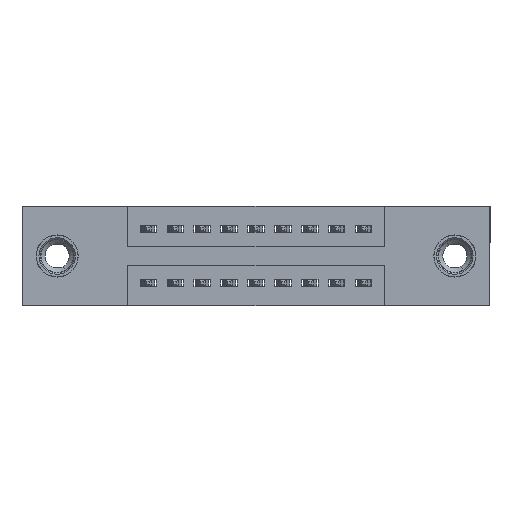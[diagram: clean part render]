
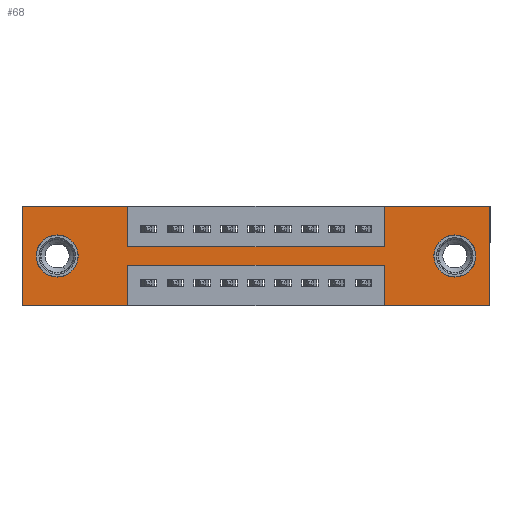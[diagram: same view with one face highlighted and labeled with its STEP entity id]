
A CAD part, front view. The second image highlights one B-rep face of the part: STEP entity #68.
In plain terms, the highlighted planar face has unit normal (0, -1, 0).
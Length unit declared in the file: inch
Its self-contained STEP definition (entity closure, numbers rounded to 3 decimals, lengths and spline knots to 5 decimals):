
#68 = ADVANCED_FACE ( 'NONE', ( #8803, #8489, #3202 ), #11013, .T. ) ;
#75 = VECTOR ( 'NONE', #6077, 39.37008 ) ;
#121 = ORIENTED_EDGE ( 'NONE', *, *, #4390, .F. ) ;
#221 = CARTESIAN_POINT ( 'NONE',  ( 1.735, 0., 0. ) ) ;
#295 = ORIENTED_EDGE ( 'NONE', *, *, #6476, .F. ) ;
#398 = ORIENTED_EDGE ( 'NONE', *, *, #9743, .F. ) ;
#426 = ORIENTED_EDGE ( 'NONE', *, *, #1014, .T. ) ;
#465 = VECTOR ( 'NONE', #7300, 39.37008 ) ;
#484 = CARTESIAN_POINT ( 'NONE',  ( 0.3925, 0., -0.15 ) ) ;
#605 = CARTESIAN_POINT ( 'NONE',  ( 0.3925, 0., 0. ) ) ;
#622 = ORIENTED_EDGE ( 'NONE', *, *, #8264, .F. ) ;
#730 = ORIENTED_EDGE ( 'NONE', *, *, #12410, .F. ) ;
#769 = AXIS2_PLACEMENT_3D ( 'NONE', #3622, #1763, #5733 ) ;
#775 = DIRECTION ( 'NONE',  ( 0., 1., 0. ) ) ;
#823 = DIRECTION ( 'NONE',  ( 0., 0., 1. ) ) ;
#894 = CIRCLE ( 'NONE', #769, 0.078 ) ;
#902 = CARTESIAN_POINT ( 'NONE',  ( 1.735, 0., -0.37 ) ) ;
#1014 = EDGE_CURVE ( 'NONE', #13647, #3405, #894, .T. ) ;
#1041 = CARTESIAN_POINT ( 'NONE',  ( 1.605, 0., -0.185 ) ) ;
#1170 = ORIENTED_EDGE ( 'NONE', *, *, #13199, .F. ) ;
#1178 = VERTEX_POINT ( 'NONE', #12595 ) ;
#1320 = DIRECTION ( 'NONE',  ( 0., 0., 1. ) ) ;
#1763 = DIRECTION ( 'NONE',  ( 0., 1., 0. ) ) ;
#1795 = DIRECTION ( 'NONE',  ( -1., 0., 0. ) ) ;
#1979 = VERTEX_POINT ( 'NONE', #3802 ) ;
#2170 = DIRECTION ( 'NONE',  ( 0., 0., -1. ) ) ;
#2199 = CARTESIAN_POINT ( 'NONE',  ( 1.3425, 0., -0.15 ) ) ;
#2228 = VECTOR ( 'NONE', #8038, 39.37008 ) ;
#2439 = EDGE_CURVE ( 'NONE', #11570, #10662, #11628, .T. ) ;
#2443 = VECTOR ( 'NONE', #3282, 39.37008 ) ;
#2457 = ORIENTED_EDGE ( 'NONE', *, *, #8968, .F. ) ;
#2541 = VERTEX_POINT ( 'NONE', #12316 ) ;
#2632 = CARTESIAN_POINT ( 'NONE',  ( 0., 0., -0.37 ) ) ;
#2906 = CARTESIAN_POINT ( 'NONE',  ( 0., 0., -0.37 ) ) ;
#2926 = DIRECTION ( 'NONE',  ( 0., 0., 1. ) ) ;
#3031 = EDGE_CURVE ( 'NONE', #1178, #9195, #13039, .T. ) ;
#3038 = VERTEX_POINT ( 'NONE', #902 ) ;
#3070 = VERTEX_POINT ( 'NONE', #221 ) ;
#3202 = FACE_OUTER_BOUND ( 'NONE', #6542, .T. ) ;
#3226 = EDGE_CURVE ( 'NONE', #9195, #5129, #10814, .T. ) ;
#3282 = DIRECTION ( 'NONE',  ( 0., 0., -1. ) ) ;
#3405 = VERTEX_POINT ( 'NONE', #11128 ) ;
#3507 = CARTESIAN_POINT ( 'NONE',  ( 0.3925, 0., -0.22 ) ) ;
#3622 = CARTESIAN_POINT ( 'NONE',  ( 1.605, 0., -0.185 ) ) ;
#3802 = CARTESIAN_POINT ( 'NONE',  ( 1.3425, 0., -0.37 ) ) ;
#3890 = ORIENTED_EDGE ( 'NONE', *, *, #10274, .F. ) ;
#3920 = VERTEX_POINT ( 'NONE', #7402 ) ;
#3952 = DIRECTION ( 'NONE',  ( -1., 0., 0. ) ) ;
#4301 = ORIENTED_EDGE ( 'NONE', *, *, #3226, .F. ) ;
#4345 = ORIENTED_EDGE ( 'NONE', *, *, #3031, .F. ) ;
#4390 = EDGE_CURVE ( 'NONE', #3920, #1178, #13333, .T. ) ;
#4460 = CARTESIAN_POINT ( 'NONE',  ( 0.3925, 0., -0.37 ) ) ;
#4507 = EDGE_CURVE ( 'NONE', #8132, #8058, #11734, .T. ) ;
#4588 = ORIENTED_EDGE ( 'NONE', *, *, #10050, .F. ) ;
#4673 = CARTESIAN_POINT ( 'NONE',  ( 0.13, 0., -0.107 ) ) ;
#4683 = CARTESIAN_POINT ( 'NONE',  ( 0., 0., 0. ) ) ;
#4693 = ORIENTED_EDGE ( 'NONE', *, *, #7794, .T. ) ;
#4987 = ORIENTED_EDGE ( 'NONE', *, *, #4507, .F. ) ;
#5129 = VERTEX_POINT ( 'NONE', #484 ) ;
#5218 = LINE ( 'NONE', #13272, #75 ) ;
#5311 = ORIENTED_EDGE ( 'NONE', *, *, #9170, .T. ) ;
#5390 = CARTESIAN_POINT ( 'NONE',  ( 0.3925, 0., 0. ) ) ;
#5636 = EDGE_LOOP ( 'NONE', ( #5311, #426 ) ) ;
#5733 = DIRECTION ( 'NONE',  ( 0., 0., -1. ) ) ;
#5920 = AXIS2_PLACEMENT_3D ( 'NONE', #7246, #775, #8296 ) ;
#6077 = DIRECTION ( 'NONE',  ( 0., 0., -1. ) ) ;
#6194 = DIRECTION ( 'NONE',  ( 0., 1., 0. ) ) ;
#6291 = ORIENTED_EDGE ( 'NONE', *, *, #2439, .T. ) ;
#6415 = LINE ( 'NONE', #10326, #6748 ) ;
#6476 = EDGE_CURVE ( 'NONE', #3038, #1979, #11042, .T. ) ;
#6542 = EDGE_LOOP ( 'NONE', ( #4987, #730, #1170, #295, #3890, #4588, #398, #622, #4301, #4345, #121, #2457 ) ) ;
#6748 = VECTOR ( 'NONE', #12352, 39.37008 ) ;
#7240 = VECTOR ( 'NONE', #823, 39.37008 ) ;
#7246 = CARTESIAN_POINT ( 'NONE',  ( 0.13, 0., -0.185 ) ) ;
#7300 = DIRECTION ( 'NONE',  ( 0., 0., -1. ) ) ;
#7369 = AXIS2_PLACEMENT_3D ( 'NONE', #2632, #11975, #12021 ) ;
#7402 = CARTESIAN_POINT ( 'NONE',  ( 0., 0., -0.37 ) ) ;
#7794 = EDGE_CURVE ( 'NONE', #10662, #11570, #10995, .T. ) ;
#8038 = DIRECTION ( 'NONE',  ( 0., 0., 1. ) ) ;
#8058 = VERTEX_POINT ( 'NONE', #4460 ) ;
#8082 = CARTESIAN_POINT ( 'NONE',  ( 1.3425, 0., 0. ) ) ;
#8132 = VERTEX_POINT ( 'NONE', #3507 ) ;
#8264 = EDGE_CURVE ( 'NONE', #5129, #9857, #11306, .T. ) ;
#8296 = DIRECTION ( 'NONE',  ( 0., 0., 1. ) ) ;
#8489 = FACE_BOUND ( 'NONE', #11355, .T. ) ;
#8540 = DIRECTION ( 'NONE',  ( 0., 1., 0. ) ) ;
#8563 = CIRCLE ( 'NONE', #11160, 0.078 ) ;
#8583 = VECTOR ( 'NONE', #12852, 39.37008 ) ;
#8584 = VECTOR ( 'NONE', #11018, 39.37008 ) ;
#8730 = VECTOR ( 'NONE', #1795, 39.37008 ) ;
#8803 = FACE_BOUND ( 'NONE', #5636, .T. ) ;
#8898 = VERTEX_POINT ( 'NONE', #8082 ) ;
#8967 = CARTESIAN_POINT ( 'NONE',  ( 0.3925, 0., -0.15 ) ) ;
#8968 = EDGE_CURVE ( 'NONE', #8058, #3920, #11757, .T. ) ;
#9170 = EDGE_CURVE ( 'NONE', #3405, #13647, #8563, .T. ) ;
#9184 = CARTESIAN_POINT ( 'NONE',  ( 0., 0., -0.37 ) ) ;
#9195 = VERTEX_POINT ( 'NONE', #5390 ) ;
#9274 = CARTESIAN_POINT ( 'NONE',  ( 0., 0., 0. ) ) ;
#9353 = CARTESIAN_POINT ( 'NONE',  ( 1.605, 0., -0.263 ) ) ;
#9496 = VECTOR ( 'NONE', #1320, 39.37008 ) ;
#9743 = EDGE_CURVE ( 'NONE', #9857, #8898, #12677, .T. ) ;
#9857 = VERTEX_POINT ( 'NONE', #2199 ) ;
#10050 = EDGE_CURVE ( 'NONE', #8898, #3070, #13629, .T. ) ;
#10274 = EDGE_CURVE ( 'NONE', #3070, #3038, #5218, .T. ) ;
#10326 = CARTESIAN_POINT ( 'NONE',  ( 0.3925, 0., -0.22 ) ) ;
#10412 = AXIS2_PLACEMENT_3D ( 'NONE', #11613, #6194, #2926 ) ;
#10662 = VERTEX_POINT ( 'NONE', #12862 ) ;
#10791 = CARTESIAN_POINT ( 'NONE',  ( 1.3425, 0., -0.37 ) ) ;
#10814 = LINE ( 'NONE', #605, #2443 ) ;
#10995 = CIRCLE ( 'NONE', #5920, 0.078 ) ;
#11013 = PLANE ( 'NONE',  #7369 ) ;
#11018 = DIRECTION ( 'NONE',  ( 1., 0., 0. ) ) ;
#11042 = LINE ( 'NONE', #9184, #12764 ) ;
#11128 = CARTESIAN_POINT ( 'NONE',  ( 1.605, 0., -0.107 ) ) ;
#11160 = AXIS2_PLACEMENT_3D ( 'NONE', #1041, #8540, #2170 ) ;
#11258 = VECTOR ( 'NONE', #12917, 39.37008 ) ;
#11306 = LINE ( 'NONE', #8967, #8584 ) ;
#11355 = EDGE_LOOP ( 'NONE', ( #6291, #4693 ) ) ;
#11570 = VERTEX_POINT ( 'NONE', #4673 ) ;
#11613 = CARTESIAN_POINT ( 'NONE',  ( 0.13, 0., -0.185 ) ) ;
#11628 = CIRCLE ( 'NONE', #10412, 0.078 ) ;
#11734 = LINE ( 'NONE', #11850, #465 ) ;
#11757 = LINE ( 'NONE', #2906, #8730 ) ;
#11850 = CARTESIAN_POINT ( 'NONE',  ( 0.3925, 0., -0.37 ) ) ;
#11975 = DIRECTION ( 'NONE',  ( 0., -1., 0. ) ) ;
#12021 = DIRECTION ( 'NONE',  ( 0., 0., -1. ) ) ;
#12179 = LINE ( 'NONE', #10791, #9496 ) ;
#12316 = CARTESIAN_POINT ( 'NONE',  ( 1.3425, 0., -0.22 ) ) ;
#12352 = DIRECTION ( 'NONE',  ( -1., 0., 0. ) ) ;
#12410 = EDGE_CURVE ( 'NONE', #2541, #8132, #6415, .T. ) ;
#12595 = CARTESIAN_POINT ( 'NONE',  ( 0., 0., 0. ) ) ;
#12677 = LINE ( 'NONE', #13470, #7240 ) ;
#12764 = VECTOR ( 'NONE', #3952, 39.37008 ) ;
#12831 = CARTESIAN_POINT ( 'NONE',  ( 0., 0., 0. ) ) ;
#12852 = DIRECTION ( 'NONE',  ( 1., 0., 0. ) ) ;
#12862 = CARTESIAN_POINT ( 'NONE',  ( 0.13, 0., -0.263 ) ) ;
#12917 = DIRECTION ( 'NONE',  ( 1., 0., 0. ) ) ;
#13039 = LINE ( 'NONE', #12831, #8583 ) ;
#13199 = EDGE_CURVE ( 'NONE', #1979, #2541, #12179, .T. ) ;
#13272 = CARTESIAN_POINT ( 'NONE',  ( 1.735, 0., 0. ) ) ;
#13333 = LINE ( 'NONE', #9274, #2228 ) ;
#13470 = CARTESIAN_POINT ( 'NONE',  ( 1.3425, 0., 0. ) ) ;
#13629 = LINE ( 'NONE', #4683, #11258 ) ;
#13647 = VERTEX_POINT ( 'NONE', #9353 ) ;
